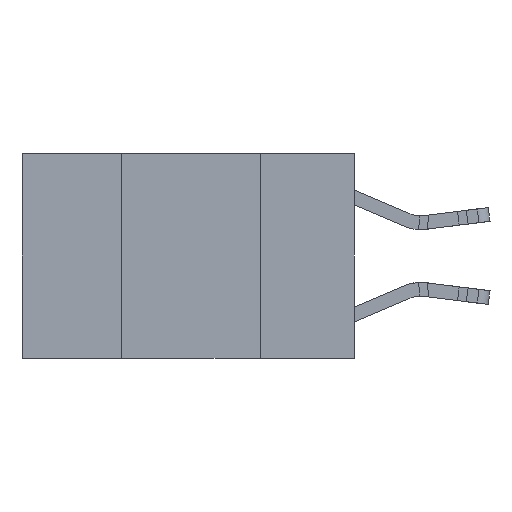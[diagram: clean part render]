
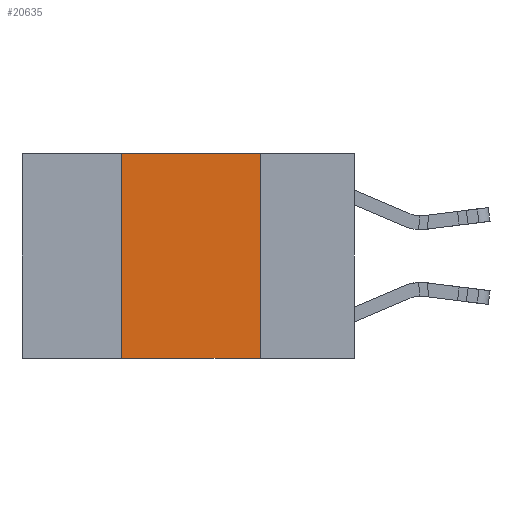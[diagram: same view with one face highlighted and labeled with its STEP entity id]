
A CAD part, left-side view. The second image highlights one B-rep face of the part: STEP entity #20635.
In plain terms, the highlighted planar face has unit normal (-1, 0, 0).
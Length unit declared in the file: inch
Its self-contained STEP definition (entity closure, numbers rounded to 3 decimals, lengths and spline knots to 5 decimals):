
#1259 = EDGE_LOOP ( 'NONE', ( #4423, #3826, #18958, #10186 ) ) ;
#1275 = VECTOR ( 'NONE', #7826, 39.37008 ) ;
#2366 = CARTESIAN_POINT ( 'NONE',  ( 0., 0.17, 0. ) ) ;
#2463 = LINE ( 'NONE', #20793, #18968 ) ;
#2620 = DIRECTION ( 'NONE',  ( 0., 0., -1. ) ) ;
#3348 = CARTESIAN_POINT ( 'NONE',  ( 0., 0.17, 0. ) ) ;
#3826 = ORIENTED_EDGE ( 'NONE', *, *, #16954, .F. ) ;
#4216 = VERTEX_POINT ( 'NONE', #2366 ) ;
#4423 = ORIENTED_EDGE ( 'NONE', *, *, #12515, .F. ) ;
#4449 = PLANE ( 'NONE',  #17767 ) ;
#4752 = DIRECTION ( 'NONE',  ( 1., 0., 0. ) ) ;
#4885 = DIRECTION ( 'NONE',  ( 0., 0., 1. ) ) ;
#5702 = LINE ( 'NONE', #28847, #1275 ) ;
#5918 = DIRECTION ( 'NONE',  ( 0., -1., 0. ) ) ;
#7151 = CARTESIAN_POINT ( 'NONE',  ( 0., 0.6, 0. ) ) ;
#7510 = EDGE_CURVE ( 'NONE', #12460, #29663, #2463, .T. ) ;
#7826 = DIRECTION ( 'NONE',  ( 0., -1., 0. ) ) ;
#8493 = LINE ( 'NONE', #17295, #27323 ) ;
#10186 = ORIENTED_EDGE ( 'NONE', *, *, #19917, .T. ) ;
#10312 = DIRECTION ( 'NONE',  ( 0., 0., -1. ) ) ;
#11017 = CARTESIAN_POINT ( 'NONE',  ( 0., 0.42, 0. ) ) ;
#11674 = VERTEX_POINT ( 'NONE', #22380 ) ;
#12290 = CARTESIAN_POINT ( 'NONE',  ( 0., 0.42, -0.37 ) ) ;
#12460 = VERTEX_POINT ( 'NONE', #12290 ) ;
#12515 = EDGE_CURVE ( 'NONE', #4216, #11674, #26501, .T. ) ;
#16954 = EDGE_CURVE ( 'NONE', #29663, #4216, #8493, .T. ) ;
#17021 = VECTOR ( 'NONE', #10312, 39.37008 ) ;
#17295 = CARTESIAN_POINT ( 'NONE',  ( 0., 0.6, 0. ) ) ;
#17767 = AXIS2_PLACEMENT_3D ( 'NONE', #7151, #4752, #2620 ) ;
#18958 = ORIENTED_EDGE ( 'NONE', *, *, #7510, .F. ) ;
#18968 = VECTOR ( 'NONE', #4885, 39.37008 ) ;
#19917 = EDGE_CURVE ( 'NONE', #12460, #11674, #5702, .T. ) ;
#20635 = ADVANCED_FACE ( 'NONE', ( #27745 ), #4449, .F. ) ;
#20793 = CARTESIAN_POINT ( 'NONE',  ( 0., 0.42, 0. ) ) ;
#22380 = CARTESIAN_POINT ( 'NONE',  ( 0., 0.17, -0.37 ) ) ;
#26501 = LINE ( 'NONE', #3348, #17021 ) ;
#27323 = VECTOR ( 'NONE', #5918, 39.37008 ) ;
#27745 = FACE_OUTER_BOUND ( 'NONE', #1259, .T. ) ;
#28847 = CARTESIAN_POINT ( 'NONE',  ( 0., 0.6, -0.37 ) ) ;
#29663 = VERTEX_POINT ( 'NONE', #11017 ) ;
